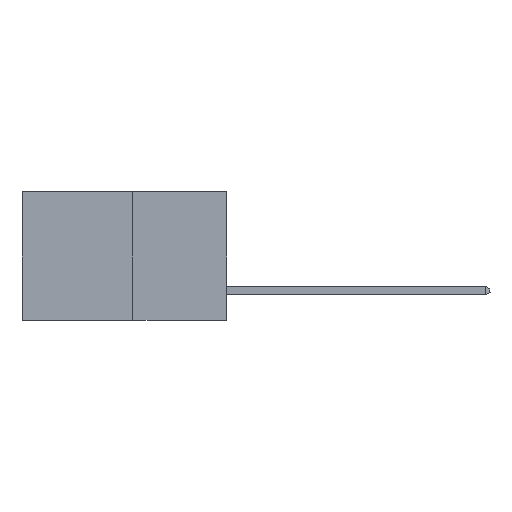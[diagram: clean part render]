
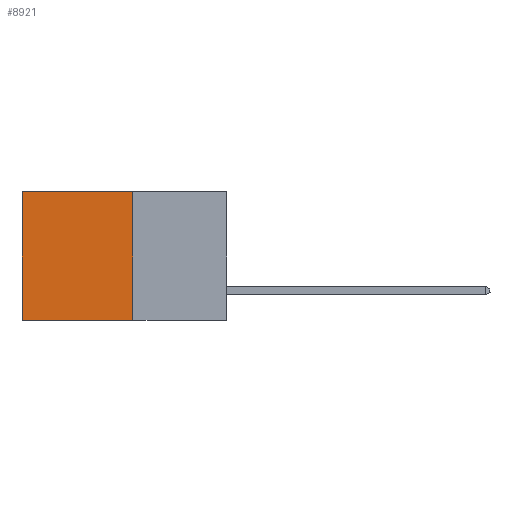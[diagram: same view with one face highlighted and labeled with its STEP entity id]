
A CAD part, left-side view. The second image highlights one B-rep face of the part: STEP entity #8921.
In plain terms, the highlighted planar face has unit normal (-1, 0, 0).
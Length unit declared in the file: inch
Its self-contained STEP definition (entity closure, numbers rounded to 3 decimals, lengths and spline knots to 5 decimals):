
#426 = CARTESIAN_POINT ( 'NONE',  ( 0.277, 0.27, -0.37 ) ) ;
#663 = ORIENTED_EDGE ( 'NONE', *, *, #11672, .T. ) ;
#680 = CARTESIAN_POINT ( 'NONE',  ( 0.277, 0.59, -0.37 ) ) ;
#807 = ORIENTED_EDGE ( 'NONE', *, *, #5000, .F. ) ;
#844 = ORIENTED_EDGE ( 'NONE', *, *, #3357, .F. ) ;
#1036 = DIRECTION ( 'NONE',  ( 0., 1., 0. ) ) ;
#1206 = ORIENTED_EDGE ( 'NONE', *, *, #13960, .T. ) ;
#2411 = VECTOR ( 'NONE', #2693, 39.37008 ) ;
#2693 = DIRECTION ( 'NONE',  ( 0., 1., 0. ) ) ;
#3357 = EDGE_CURVE ( 'NONE', #7203, #8401, #3741, .T. ) ;
#3741 = LINE ( 'NONE', #426, #12171 ) ;
#3849 = EDGE_LOOP ( 'NONE', ( #1206, #807, #844, #663 ) ) ;
#3900 = CARTESIAN_POINT ( 'NONE',  ( 0.277, 0.27, -0.37 ) ) ;
#4764 = VERTEX_POINT ( 'NONE', #8374 ) ;
#5000 = EDGE_CURVE ( 'NONE', #8401, #5854, #13992, .T. ) ;
#5419 = CARTESIAN_POINT ( 'NONE',  ( 0.277, 0.27, -0.37 ) ) ;
#5666 = DIRECTION ( 'NONE',  ( 0., 0., -1. ) ) ;
#5854 = VERTEX_POINT ( 'NONE', #680 ) ;
#5907 = CARTESIAN_POINT ( 'NONE',  ( 0.277, 0.27, -0.37 ) ) ;
#6842 = FACE_OUTER_BOUND ( 'NONE', #3849, .T. ) ;
#7070 = DIRECTION ( 'NONE',  ( 0., 0., -1. ) ) ;
#7126 = DIRECTION ( 'NONE',  ( 0., 0., -1. ) ) ;
#7203 = VERTEX_POINT ( 'NONE', #8474 ) ;
#8202 = VECTOR ( 'NONE', #1036, 39.37008 ) ;
#8374 = CARTESIAN_POINT ( 'NONE',  ( 0.277, 0.59, 0. ) ) ;
#8401 = VERTEX_POINT ( 'NONE', #3900 ) ;
#8474 = CARTESIAN_POINT ( 'NONE',  ( 0.277, 0.27, 0. ) ) ;
#8917 = CARTESIAN_POINT ( 'NONE',  ( 0.277, 0.59, -0.37 ) ) ;
#8921 = ADVANCED_FACE ( 'NONE', ( #6842 ), #11394, .F. ) ;
#10328 = LINE ( 'NONE', #8917, #12917 ) ;
#11177 = LINE ( 'NONE', #11465, #2411 ) ;
#11394 = PLANE ( 'NONE',  #11421 ) ;
#11421 = AXIS2_PLACEMENT_3D ( 'NONE', #5907, #13581, #7070 ) ;
#11465 = CARTESIAN_POINT ( 'NONE',  ( 0.277, 0.27, 0. ) ) ;
#11672 = EDGE_CURVE ( 'NONE', #7203, #4764, #11177, .T. ) ;
#12171 = VECTOR ( 'NONE', #7126, 39.37008 ) ;
#12917 = VECTOR ( 'NONE', #5666, 39.37008 ) ;
#13581 = DIRECTION ( 'NONE',  ( 1., 0., 0. ) ) ;
#13960 = EDGE_CURVE ( 'NONE', #4764, #5854, #10328, .T. ) ;
#13992 = LINE ( 'NONE', #5419, #8202 ) ;
